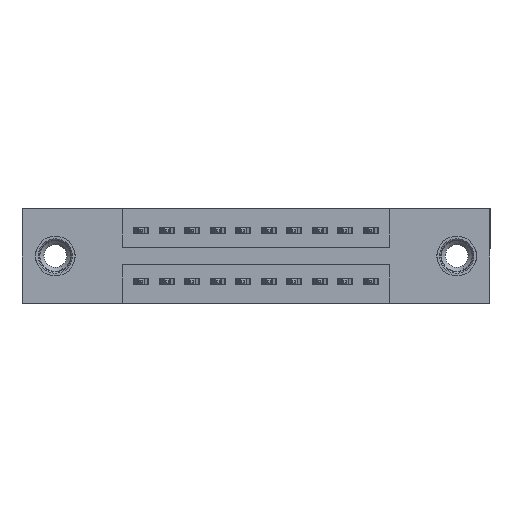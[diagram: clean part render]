
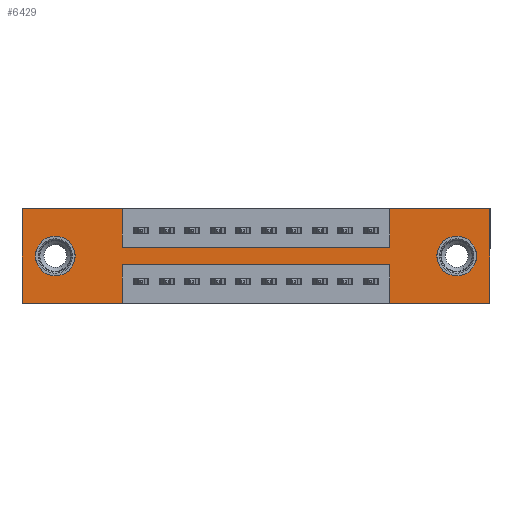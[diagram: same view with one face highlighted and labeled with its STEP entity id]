
A CAD part, front view. The second image highlights one B-rep face of the part: STEP entity #6429.
In plain terms, the highlighted planar face has unit normal (0, -1, 0).
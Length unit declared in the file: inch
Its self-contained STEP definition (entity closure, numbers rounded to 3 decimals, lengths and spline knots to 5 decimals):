
#430 = VERTEX_POINT ( 'NONE', #11572 ) ;
#437 = VERTEX_POINT ( 'NONE', #12017 ) ;
#447 = DIRECTION ( 'NONE',  ( 1., 0., 0. ) ) ;
#536 = DIRECTION ( 'NONE',  ( 0., 0., -1. ) ) ;
#677 = ORIENTED_EDGE ( 'NONE', *, *, #10394, .T. ) ;
#905 = CARTESIAN_POINT ( 'NONE',  ( 1.705, 0., -0.107 ) ) ;
#1008 = VECTOR ( 'NONE', #12213, 39.37008 ) ;
#1026 = AXIS2_PLACEMENT_3D ( 'NONE', #4242, #8562, #10216 ) ;
#1155 = ORIENTED_EDGE ( 'NONE', *, *, #13812, .T. ) ;
#1190 = CARTESIAN_POINT ( 'NONE',  ( 0., 0., -0.37 ) ) ;
#1332 = ORIENTED_EDGE ( 'NONE', *, *, #1909, .T. ) ;
#1650 = CARTESIAN_POINT ( 'NONE',  ( 1.4425, 0., 0. ) ) ;
#1664 = VERTEX_POINT ( 'NONE', #12093 ) ;
#1707 = VECTOR ( 'NONE', #8746, 39.37008 ) ;
#1720 = LINE ( 'NONE', #3625, #9101 ) ;
#1756 = EDGE_CURVE ( 'NONE', #15257, #8604, #5292, .T. ) ;
#1875 = ORIENTED_EDGE ( 'NONE', *, *, #9327, .F. ) ;
#1886 = LINE ( 'NONE', #15927, #5048 ) ;
#1909 = EDGE_CURVE ( 'NONE', #437, #13641, #16913, .T. ) ;
#2235 = EDGE_CURVE ( 'NONE', #7598, #13509, #4860, .T. ) ;
#2288 = CARTESIAN_POINT ( 'NONE',  ( 0., 0., -0.37 ) ) ;
#2432 = LINE ( 'NONE', #1650, #15825 ) ;
#2600 = CARTESIAN_POINT ( 'NONE',  ( 1.4425, 0., -0.37 ) ) ;
#2862 = AXIS2_PLACEMENT_3D ( 'NONE', #13623, #5892, #14894 ) ;
#3010 = DIRECTION ( 'NONE',  ( 0., 0., 1. ) ) ;
#3029 = DIRECTION ( 'NONE',  ( -1., 0., 0. ) ) ;
#3072 = ORIENTED_EDGE ( 'NONE', *, *, #7520, .F. ) ;
#3138 = EDGE_CURVE ( 'NONE', #3623, #7708, #3571, .T. ) ;
#3400 = ORIENTED_EDGE ( 'NONE', *, *, #12645, .F. ) ;
#3571 = CIRCLE ( 'NONE', #1026, 0.078 ) ;
#3606 = ORIENTED_EDGE ( 'NONE', *, *, #3138, .T. ) ;
#3623 = VERTEX_POINT ( 'NONE', #4971 ) ;
#3625 = CARTESIAN_POINT ( 'NONE',  ( 1.4425, 0., -0.37 ) ) ;
#4036 = CARTESIAN_POINT ( 'NONE',  ( 1.705, 0., -0.185 ) ) ;
#4144 = CARTESIAN_POINT ( 'NONE',  ( 0.13, 0., -0.263 ) ) ;
#4242 = CARTESIAN_POINT ( 'NONE',  ( 1.705, 0., -0.185 ) ) ;
#4364 = ORIENTED_EDGE ( 'NONE', *, *, #7736, .F. ) ;
#4775 = EDGE_CURVE ( 'NONE', #16165, #7598, #15677, .T. ) ;
#4860 = LINE ( 'NONE', #14295, #15146 ) ;
#4971 = CARTESIAN_POINT ( 'NONE',  ( 1.705, 0., -0.263 ) ) ;
#5017 = VECTOR ( 'NONE', #5337, 39.37008 ) ;
#5046 = VECTOR ( 'NONE', #447, 39.37008 ) ;
#5048 = VECTOR ( 'NONE', #12157, 39.37008 ) ;
#5051 = DIRECTION ( 'NONE',  ( 0., -1., 0. ) ) ;
#5112 = CARTESIAN_POINT ( 'NONE',  ( 0., 0., 0. ) ) ;
#5292 = LINE ( 'NONE', #15368, #1707 ) ;
#5337 = DIRECTION ( 'NONE',  ( -1., 0., 0. ) ) ;
#5406 = DIRECTION ( 'NONE',  ( 0., 0., -1. ) ) ;
#5493 = EDGE_LOOP ( 'NONE', ( #677, #3606 ) ) ;
#5540 = VERTEX_POINT ( 'NONE', #10827 ) ;
#5578 = FACE_BOUND ( 'NONE', #5493, .T. ) ;
#5756 = CARTESIAN_POINT ( 'NONE',  ( 1.4425, 0., -0.22 ) ) ;
#5892 = DIRECTION ( 'NONE',  ( 0., 1., 0. ) ) ;
#5910 = VERTEX_POINT ( 'NONE', #16625 ) ;
#6429 = ADVANCED_FACE ( 'NONE', ( #5578, #8962, #15826 ), #10177, .T. ) ;
#6470 = DIRECTION ( 'NONE',  ( 0., 0., 1. ) ) ;
#6751 = VECTOR ( 'NONE', #3029, 39.37008 ) ;
#6859 = EDGE_CURVE ( 'NONE', #8604, #11656, #16594, .T. ) ;
#7147 = CARTESIAN_POINT ( 'NONE',  ( 0.3925, 0., -0.22 ) ) ;
#7440 = VERTEX_POINT ( 'NONE', #5756 ) ;
#7520 = EDGE_CURVE ( 'NONE', #7440, #1664, #8909, .T. ) ;
#7598 = VERTEX_POINT ( 'NONE', #9978 ) ;
#7708 = VERTEX_POINT ( 'NONE', #905 ) ;
#7736 = EDGE_CURVE ( 'NONE', #11656, #7440, #1720, .T. ) ;
#8272 = CARTESIAN_POINT ( 'NONE',  ( 0., 0., 0. ) ) ;
#8424 = DIRECTION ( 'NONE',  ( -1., 0., 0. ) ) ;
#8478 = CARTESIAN_POINT ( 'NONE',  ( 0.3925, 0., -0.37 ) ) ;
#8562 = DIRECTION ( 'NONE',  ( 0., 1., 0. ) ) ;
#8604 = VERTEX_POINT ( 'NONE', #16113 ) ;
#8746 = DIRECTION ( 'NONE',  ( 0., 0., -1. ) ) ;
#8795 = VECTOR ( 'NONE', #536, 39.37008 ) ;
#8909 = LINE ( 'NONE', #7147, #11590 ) ;
#8962 = FACE_BOUND ( 'NONE', #9719, .T. ) ;
#9046 = DIRECTION ( 'NONE',  ( 1., 0., 0. ) ) ;
#9101 = VECTOR ( 'NONE', #11744, 39.37008 ) ;
#9130 = DIRECTION ( 'NONE',  ( 0., 0., 1. ) ) ;
#9224 = DIRECTION ( 'NONE',  ( 0., 1., 0. ) ) ;
#9327 = EDGE_CURVE ( 'NONE', #5540, #5910, #11928, .T. ) ;
#9719 = EDGE_LOOP ( 'NONE', ( #1332, #1155 ) ) ;
#9783 = CARTESIAN_POINT ( 'NONE',  ( 0.13, 0., -0.185 ) ) ;
#9784 = ORIENTED_EDGE ( 'NONE', *, *, #4775, .F. ) ;
#9960 = AXIS2_PLACEMENT_3D ( 'NONE', #4036, #13137, #5406 ) ;
#9978 = CARTESIAN_POINT ( 'NONE',  ( 0., 0., -0.37 ) ) ;
#10125 = ORIENTED_EDGE ( 'NONE', *, *, #14323, .F. ) ;
#10177 = PLANE ( 'NONE',  #11238 ) ;
#10216 = DIRECTION ( 'NONE',  ( 0., 0., -1. ) ) ;
#10286 = AXIS2_PLACEMENT_3D ( 'NONE', #9783, #9224, #9130 ) ;
#10394 = EDGE_CURVE ( 'NONE', #7708, #3623, #11327, .T. ) ;
#10626 = CARTESIAN_POINT ( 'NONE',  ( 0.3925, 0., -0.37 ) ) ;
#10827 = CARTESIAN_POINT ( 'NONE',  ( 0.3925, 0., -0.15 ) ) ;
#11032 = CARTESIAN_POINT ( 'NONE',  ( 0.3925, 0., -0.15 ) ) ;
#11238 = AXIS2_PLACEMENT_3D ( 'NONE', #2288, #5051, #14071 ) ;
#11327 = CIRCLE ( 'NONE', #9960, 0.078 ) ;
#11534 = LINE ( 'NONE', #8272, #1008 ) ;
#11572 = CARTESIAN_POINT ( 'NONE',  ( 0.3925, 0., 0. ) ) ;
#11590 = VECTOR ( 'NONE', #8424, 39.37008 ) ;
#11656 = VERTEX_POINT ( 'NONE', #2600 ) ;
#11744 = DIRECTION ( 'NONE',  ( 0., 0., 1. ) ) ;
#11769 = CARTESIAN_POINT ( 'NONE',  ( 0., 0., 0. ) ) ;
#11867 = VERTEX_POINT ( 'NONE', #13315 ) ;
#11928 = LINE ( 'NONE', #11032, #5046 ) ;
#11994 = ORIENTED_EDGE ( 'NONE', *, *, #2235, .F. ) ;
#12017 = CARTESIAN_POINT ( 'NONE',  ( 0.13, 0., -0.107 ) ) ;
#12093 = CARTESIAN_POINT ( 'NONE',  ( 0.3925, 0., -0.22 ) ) ;
#12157 = DIRECTION ( 'NONE',  ( 0., 0., -1. ) ) ;
#12191 = ORIENTED_EDGE ( 'NONE', *, *, #6859, .F. ) ;
#12213 = DIRECTION ( 'NONE',  ( 1., 0., 0. ) ) ;
#12253 = VECTOR ( 'NONE', #9046, 39.37008 ) ;
#12447 = EDGE_CURVE ( 'NONE', #11867, #15257, #16030, .T. ) ;
#12645 = EDGE_CURVE ( 'NONE', #5910, #11867, #2432, .T. ) ;
#12687 = LINE ( 'NONE', #8478, #8795 ) ;
#13014 = ORIENTED_EDGE ( 'NONE', *, *, #14370, .F. ) ;
#13137 = DIRECTION ( 'NONE',  ( 0., 1., 0. ) ) ;
#13315 = CARTESIAN_POINT ( 'NONE',  ( 1.4425, 0., 0. ) ) ;
#13509 = VERTEX_POINT ( 'NONE', #5112 ) ;
#13623 = CARTESIAN_POINT ( 'NONE',  ( 0.13, 0., -0.185 ) ) ;
#13641 = VERTEX_POINT ( 'NONE', #4144 ) ;
#13697 = ORIENTED_EDGE ( 'NONE', *, *, #1756, .F. ) ;
#13812 = EDGE_CURVE ( 'NONE', #13641, #437, #16373, .T. ) ;
#14071 = DIRECTION ( 'NONE',  ( 0., 0., -1. ) ) ;
#14295 = CARTESIAN_POINT ( 'NONE',  ( 0., 0., 0. ) ) ;
#14323 = EDGE_CURVE ( 'NONE', #430, #5540, #1886, .T. ) ;
#14370 = EDGE_CURVE ( 'NONE', #13509, #430, #11534, .T. ) ;
#14894 = DIRECTION ( 'NONE',  ( 0., 0., 1. ) ) ;
#15146 = VECTOR ( 'NONE', #6470, 39.37008 ) ;
#15220 = CARTESIAN_POINT ( 'NONE',  ( 1.835, 0., 0. ) ) ;
#15257 = VERTEX_POINT ( 'NONE', #15220 ) ;
#15368 = CARTESIAN_POINT ( 'NONE',  ( 1.835, 0., 0. ) ) ;
#15537 = ORIENTED_EDGE ( 'NONE', *, *, #12447, .F. ) ;
#15677 = LINE ( 'NONE', #1190, #5017 ) ;
#15699 = EDGE_CURVE ( 'NONE', #1664, #16165, #12687, .T. ) ;
#15825 = VECTOR ( 'NONE', #3010, 39.37008 ) ;
#15826 = FACE_OUTER_BOUND ( 'NONE', #16144, .T. ) ;
#15927 = CARTESIAN_POINT ( 'NONE',  ( 0.3925, 0., 0. ) ) ;
#16030 = LINE ( 'NONE', #11769, #12253 ) ;
#16054 = CARTESIAN_POINT ( 'NONE',  ( 0., 0., -0.37 ) ) ;
#16113 = CARTESIAN_POINT ( 'NONE',  ( 1.835, 0., -0.37 ) ) ;
#16144 = EDGE_LOOP ( 'NONE', ( #16609, #3072, #4364, #12191, #13697, #15537, #3400, #1875, #10125, #13014, #11994, #9784 ) ) ;
#16165 = VERTEX_POINT ( 'NONE', #10626 ) ;
#16373 = CIRCLE ( 'NONE', #2862, 0.078 ) ;
#16594 = LINE ( 'NONE', #16054, #6751 ) ;
#16609 = ORIENTED_EDGE ( 'NONE', *, *, #15699, .F. ) ;
#16625 = CARTESIAN_POINT ( 'NONE',  ( 1.4425, 0., -0.15 ) ) ;
#16913 = CIRCLE ( 'NONE', #10286, 0.078 ) ;
